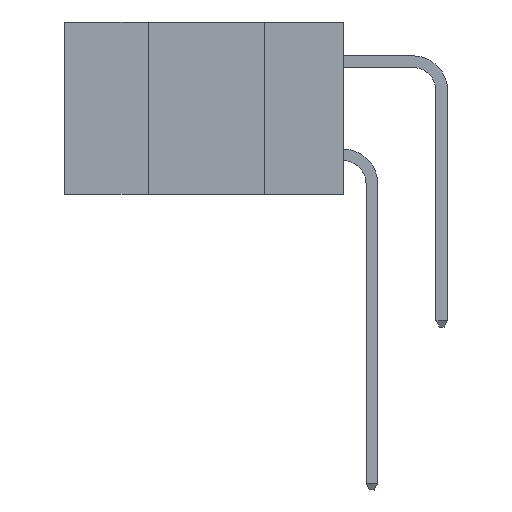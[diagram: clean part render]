
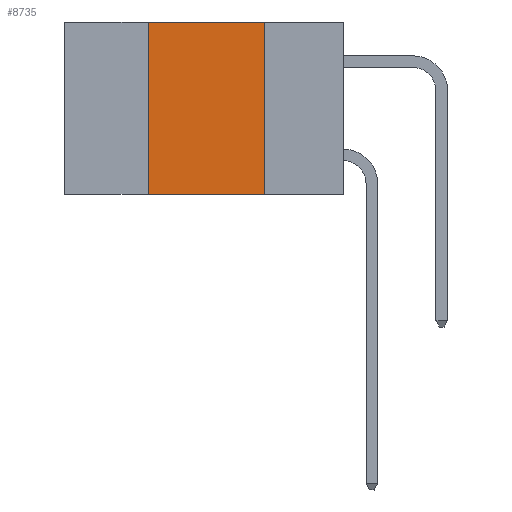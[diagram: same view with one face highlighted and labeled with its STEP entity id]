
A CAD part, left-side view. The second image highlights one B-rep face of the part: STEP entity #8735.
In plain terms, the highlighted planar face has unit normal (-1, 0, 0).
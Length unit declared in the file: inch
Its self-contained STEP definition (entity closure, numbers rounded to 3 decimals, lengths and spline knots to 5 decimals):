
#442 = CARTESIAN_POINT ( 'NONE',  ( 0., 0.42, 0. ) ) ;
#637 = EDGE_CURVE ( 'NONE', #28404, #10111, #22000, .T. ) ;
#970 = CARTESIAN_POINT ( 'NONE',  ( 0., 0.17, 0. ) ) ;
#2156 = VECTOR ( 'NONE', #24064, 39.37008 ) ;
#2993 = LINE ( 'NONE', #3089, #2156 ) ;
#3089 = CARTESIAN_POINT ( 'NONE',  ( 0., 0.6, -0.37 ) ) ;
#8735 = ADVANCED_FACE ( 'NONE', ( #9748 ), #10394, .F. ) ;
#9706 = AXIS2_PLACEMENT_3D ( 'NONE', #33731, #28679, #13014 ) ;
#9748 = FACE_OUTER_BOUND ( 'NONE', #24063, .T. ) ;
#9814 = LINE ( 'NONE', #24706, #22982 ) ;
#10111 = VERTEX_POINT ( 'NONE', #26215 ) ;
#10394 = PLANE ( 'NONE',  #9706 ) ;
#11651 = EDGE_CURVE ( 'NONE', #28404, #25333, #2993, .T. ) ;
#11783 = VERTEX_POINT ( 'NONE', #970 ) ;
#12297 = ORIENTED_EDGE ( 'NONE', *, *, #14651, .F. ) ;
#13014 = DIRECTION ( 'NONE',  ( 0., 0., -1. ) ) ;
#13102 = DIRECTION ( 'NONE',  ( 0., 0., 1. ) ) ;
#13920 = ORIENTED_EDGE ( 'NONE', *, *, #637, .F. ) ;
#14142 = CARTESIAN_POINT ( 'NONE',  ( 0., 0.17, 0. ) ) ;
#14651 = EDGE_CURVE ( 'NONE', #10111, #11783, #9814, .T. ) ;
#14989 = VECTOR ( 'NONE', #13102, 39.37008 ) ;
#18795 = EDGE_CURVE ( 'NONE', #11783, #25333, #26867, .T. ) ;
#22000 = LINE ( 'NONE', #442, #14989 ) ;
#22982 = VECTOR ( 'NONE', #27318, 39.37008 ) ;
#23397 = ORIENTED_EDGE ( 'NONE', *, *, #11651, .T. ) ;
#24063 = EDGE_LOOP ( 'NONE', ( #25416, #12297, #13920, #23397 ) ) ;
#24064 = DIRECTION ( 'NONE',  ( 0., -1., 0. ) ) ;
#24706 = CARTESIAN_POINT ( 'NONE',  ( 0., 0.6, 0. ) ) ;
#25333 = VERTEX_POINT ( 'NONE', #33792 ) ;
#25416 = ORIENTED_EDGE ( 'NONE', *, *, #18795, .F. ) ;
#26215 = CARTESIAN_POINT ( 'NONE',  ( 0., 0.42, 0. ) ) ;
#26867 = LINE ( 'NONE', #14142, #32889 ) ;
#27318 = DIRECTION ( 'NONE',  ( 0., -1., 0. ) ) ;
#27336 = CARTESIAN_POINT ( 'NONE',  ( 0., 0.42, -0.37 ) ) ;
#28404 = VERTEX_POINT ( 'NONE', #27336 ) ;
#28679 = DIRECTION ( 'NONE',  ( 1., 0., 0. ) ) ;
#29765 = DIRECTION ( 'NONE',  ( 0., 0., -1. ) ) ;
#32889 = VECTOR ( 'NONE', #29765, 39.37008 ) ;
#33731 = CARTESIAN_POINT ( 'NONE',  ( 0., 0.6, 0. ) ) ;
#33792 = CARTESIAN_POINT ( 'NONE',  ( 0., 0.17, -0.37 ) ) ;
